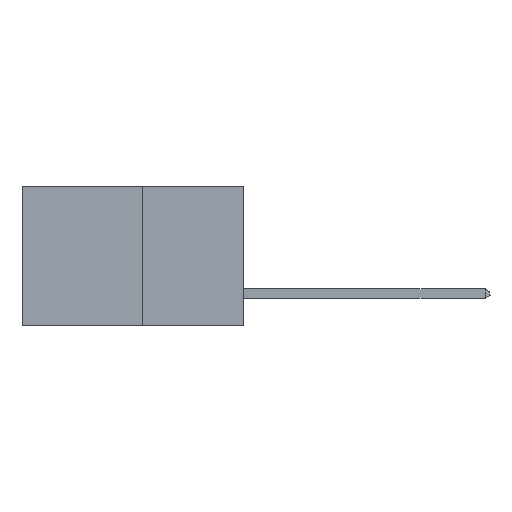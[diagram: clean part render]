
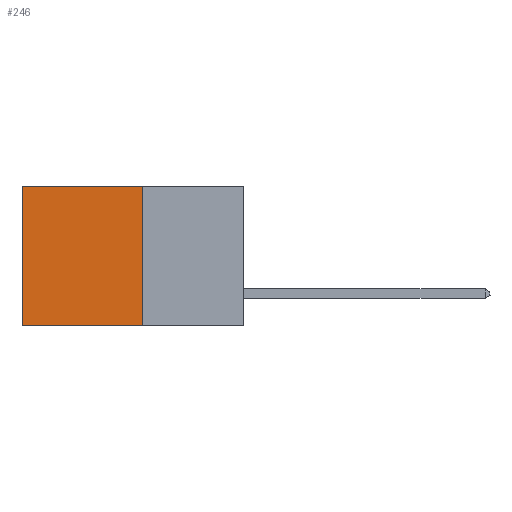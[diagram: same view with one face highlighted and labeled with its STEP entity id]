
A CAD part, left-side view. The second image highlights one B-rep face of the part: STEP entity #246.
In plain terms, the highlighted planar face has unit normal (-1, 0, 0).
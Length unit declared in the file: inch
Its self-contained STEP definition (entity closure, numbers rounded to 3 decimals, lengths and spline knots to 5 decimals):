
#246 = ADVANCED_FACE ( 'NONE', ( #591 ), #1478, .F. ) ;
#591 = FACE_OUTER_BOUND ( 'NONE', #8711, .T. ) ;
#595 = VERTEX_POINT ( 'NONE', #9482 ) ;
#1315 = CARTESIAN_POINT ( 'NONE',  ( 0.277, 0.27, 0. ) ) ;
#1478 = PLANE ( 'NONE',  #7823 ) ;
#1542 = DIRECTION ( 'NONE',  ( 0., 1., 0. ) ) ;
#1721 = CARTESIAN_POINT ( 'NONE',  ( 0.277, 0.27, -0.37 ) ) ;
#1882 = EDGE_CURVE ( 'NONE', #595, #7062, #3486, .T. ) ;
#2773 = CARTESIAN_POINT ( 'NONE',  ( 0.277, 0.27, -0.37 ) ) ;
#3080 = LINE ( 'NONE', #6267, #7825 ) ;
#3486 = LINE ( 'NONE', #12195, #10909 ) ;
#4223 = DIRECTION ( 'NONE',  ( 0., 0., -1. ) ) ;
#4477 = DIRECTION ( 'NONE',  ( 0., 0., -1. ) ) ;
#4482 = CARTESIAN_POINT ( 'NONE',  ( 0.277, 0.27, -0.37 ) ) ;
#4665 = EDGE_CURVE ( 'NONE', #9199, #8463, #11409, .T. ) ;
#5245 = EDGE_CURVE ( 'NONE', #9199, #595, #3080, .T. ) ;
#6019 = EDGE_CURVE ( 'NONE', #8463, #7062, #8929, .T. ) ;
#6267 = CARTESIAN_POINT ( 'NONE',  ( 0.277, 0.27, 0. ) ) ;
#6286 = DIRECTION ( 'NONE',  ( 0., 1., 0. ) ) ;
#6413 = ORIENTED_EDGE ( 'NONE', *, *, #1882, .T. ) ;
#6441 = CARTESIAN_POINT ( 'NONE',  ( 0.277, 0.59, -0.37 ) ) ;
#6508 = VECTOR ( 'NONE', #1542, 39.37008 ) ;
#6612 = ORIENTED_EDGE ( 'NONE', *, *, #6019, .F. ) ;
#6640 = ORIENTED_EDGE ( 'NONE', *, *, #4665, .F. ) ;
#6692 = ORIENTED_EDGE ( 'NONE', *, *, #5245, .T. ) ;
#7062 = VERTEX_POINT ( 'NONE', #6441 ) ;
#7823 = AXIS2_PLACEMENT_3D ( 'NONE', #1721, #10157, #4223 ) ;
#7825 = VECTOR ( 'NONE', #6286, 39.37008 ) ;
#8197 = CARTESIAN_POINT ( 'NONE',  ( 0.277, 0.27, -0.37 ) ) ;
#8463 = VERTEX_POINT ( 'NONE', #4482 ) ;
#8672 = VECTOR ( 'NONE', #4477, 39.37008 ) ;
#8683 = DIRECTION ( 'NONE',  ( 0., 0., -1. ) ) ;
#8711 = EDGE_LOOP ( 'NONE', ( #6413, #6612, #6640, #6692 ) ) ;
#8929 = LINE ( 'NONE', #2773, #6508 ) ;
#9199 = VERTEX_POINT ( 'NONE', #1315 ) ;
#9482 = CARTESIAN_POINT ( 'NONE',  ( 0.277, 0.59, 0. ) ) ;
#10157 = DIRECTION ( 'NONE',  ( 1., 0., 0. ) ) ;
#10909 = VECTOR ( 'NONE', #8683, 39.37008 ) ;
#11409 = LINE ( 'NONE', #8197, #8672 ) ;
#12195 = CARTESIAN_POINT ( 'NONE',  ( 0.277, 0.59, -0.37 ) ) ;
